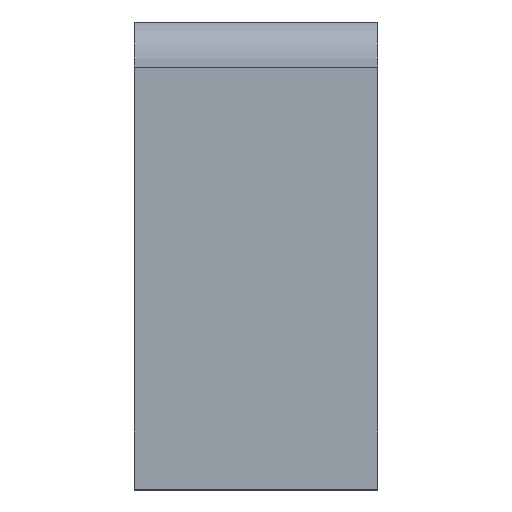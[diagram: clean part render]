
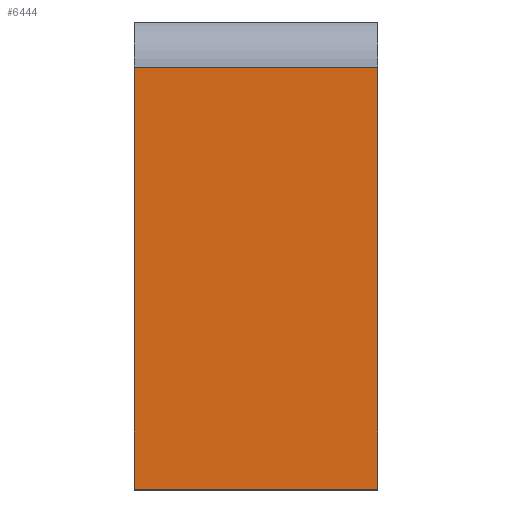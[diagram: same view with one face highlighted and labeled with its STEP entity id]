
A CAD part, top view. The second image highlights one B-rep face of the part: STEP entity #6444.
In plain terms, the highlighted planar face has unit normal (0, 0, 1).
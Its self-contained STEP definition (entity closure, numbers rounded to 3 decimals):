
#808=FACE_OUTER_BOUND('',#1148,.T.);
#1148=EDGE_LOOP('',(#5887,#5888,#5889,#5890));
#1784=LINE('',#11531,#2430);
#1786=LINE('',#11537,#2432);
#1787=LINE('',#11540,#2433);
#1788=LINE('',#11541,#2434);
#2430=VECTOR('',#7752,10.);
#2432=VECTOR('',#7758,2.11);
#2433=VECTOR('',#7763,10.);
#2434=VECTOR('',#7764,10.);
#3073=VERTEX_POINT('',#11528);
#3074=VERTEX_POINT('',#11530);
#3075=VERTEX_POINT('',#11534);
#3076=VERTEX_POINT('',#11536);
#4016=EDGE_CURVE('',#3074,#3073,#1784,.T.);
#4019=EDGE_CURVE('',#3075,#3076,#1786,.T.);
#4021=EDGE_CURVE('',#3075,#3074,#1787,.T.);
#4022=EDGE_CURVE('',#3073,#3076,#1788,.T.);
#5887=ORIENTED_EDGE('',*,*,#4019,.F.);
#5888=ORIENTED_EDGE('',*,*,#4021,.T.);
#5889=ORIENTED_EDGE('',*,*,#4016,.T.);
#5890=ORIENTED_EDGE('',*,*,#4022,.T.);
#6115=PLANE('',#6684);
#6444=ADVANCED_FACE('',(#808),#6115,.T.);
#6684=AXIS2_PLACEMENT_3D('',#11539,#7761,#7762);
#7752=DIRECTION('',(1.,0.,0.));
#7758=DIRECTION('',(1.,0.,0.));
#7761=DIRECTION('center_axis',(0.,0.,
1.));
#7762=DIRECTION('ref_axis',(0.,-1.,0.));
#7763=DIRECTION('',(0.,-1.,0.));
#7764=DIRECTION('',(0.,1.,0.));
#11528=CARTESIAN_POINT('',(-44.642,66.338,14.913));
#11530=CARTESIAN_POINT('',(-59.642,66.338,14.913));
#11531=CARTESIAN_POINT('',(-62.642,66.338,14.913));
#11534=CARTESIAN_POINT('',(-59.642,92.351,14.913));
#11536=CARTESIAN_POINT('',(-44.642,92.351,14.913));
#11537=CARTESIAN_POINT('',(-62.642,92.351,14.913));
#11539=CARTESIAN_POINT('Origin',(-62.642,86.338,14.913));
#11540=CARTESIAN_POINT('',(-59.642,86.338,14.913));
#11541=CARTESIAN_POINT('',(-44.642,86.338,14.913));
